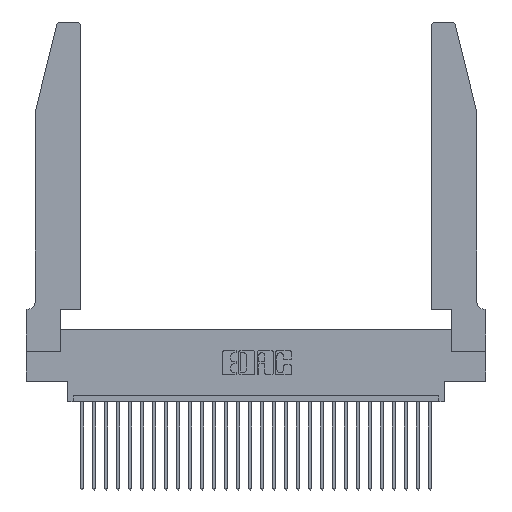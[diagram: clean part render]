
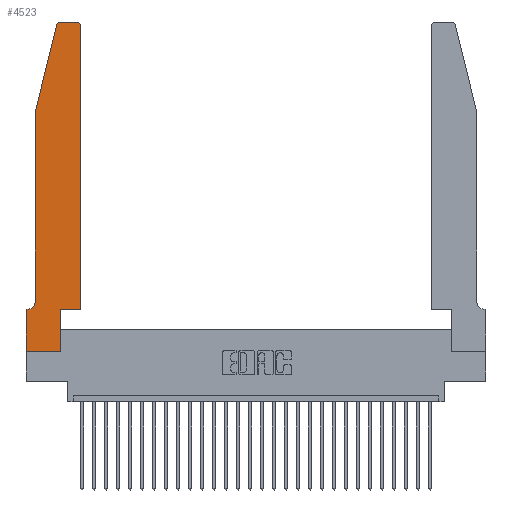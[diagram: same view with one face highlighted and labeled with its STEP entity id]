
A CAD part, top view. The second image highlights one B-rep face of the part: STEP entity #4523.
In plain terms, the highlighted planar face has unit normal (0, 0, 1).
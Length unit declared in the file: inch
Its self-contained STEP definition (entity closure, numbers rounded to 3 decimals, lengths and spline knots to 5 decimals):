
#309 = VECTOR ( 'NONE', #21141, 39.37008 ) ;
#539 = VECTOR ( 'NONE', #13087, 39.37008 ) ;
#681 = DIRECTION ( 'NONE',  ( 1., 0., 0. ) ) ;
#778 = LINE ( 'NONE', #23107, #18697 ) ;
#829 = CARTESIAN_POINT ( 'NONE',  ( 0.0755, 2., 0.37 ) ) ;
#947 = ORIENTED_EDGE ( 'NONE', *, *, #22796, .T. ) ;
#1176 = CARTESIAN_POINT ( 'NONE',  ( 0., 0.35, 0.37 ) ) ;
#1369 = VERTEX_POINT ( 'NONE', #12878 ) ;
#1539 = DIRECTION ( 'NONE',  ( 0., 1., 0. ) ) ;
#2335 = VERTEX_POINT ( 'NONE', #19658 ) ;
#2676 = DIRECTION ( 'NONE',  ( -1., 0., 0. ) ) ;
#2739 = EDGE_CURVE ( 'NONE', #14284, #28371, #19319, .T. ) ;
#2931 = CARTESIAN_POINT ( 'NONE',  ( 0.284, 2.72, 0.37 ) ) ;
#3050 = CARTESIAN_POINT ( 'NONE',  ( 0., 0., 0.37 ) ) ;
#3815 = CIRCLE ( 'NONE', #20481, 0.03 ) ;
#4523 = ADVANCED_FACE ( 'NONE', ( #9105 ), #25926, .T. ) ;
#4568 = ORIENTED_EDGE ( 'NONE', *, *, #15418, .T. ) ;
#4614 = ORIENTED_EDGE ( 'NONE', *, *, #2739, .T. ) ;
#6243 = VERTEX_POINT ( 'NONE', #11317 ) ;
#6420 = CARTESIAN_POINT ( 'NONE',  ( 0., 0., 0.37 ) ) ;
#6519 = LINE ( 'NONE', #12882, #539 ) ;
#6529 = VERTEX_POINT ( 'NONE', #8153 ) ;
#6826 = VERTEX_POINT ( 'NONE', #20742 ) ;
#7390 = DIRECTION ( 'NONE',  ( 0., 1., 0. ) ) ;
#7503 = VECTOR ( 'NONE', #20875, 39.37008 ) ;
#7656 = CIRCLE ( 'NONE', #19356, 0.07 ) ;
#7717 = DIRECTION ( 'NONE',  ( 1., 0., 0. ) ) ;
#8153 = CARTESIAN_POINT ( 'NONE',  ( 0.4505, 0.35, 0.37 ) ) ;
#8216 = DIRECTION ( 'NONE',  ( 0., 0., 1. ) ) ;
#8703 = CARTESIAN_POINT ( 'NONE',  ( 0.2605, 2.75, 0.37 ) ) ;
#9105 = FACE_OUTER_BOUND ( 'NONE', #18436, .T. ) ;
#9528 = EDGE_CURVE ( 'NONE', #6243, #6529, #22151, .T. ) ;
#9641 = EDGE_CURVE ( 'NONE', #1369, #19154, #17126, .T. ) ;
#9747 = ORIENTED_EDGE ( 'NONE', *, *, #21674, .T. ) ;
#9789 = LINE ( 'NONE', #12009, #13646 ) ;
#10173 = CARTESIAN_POINT ( 'NONE',  ( 0.0755, 2., 0.37 ) ) ;
#10863 = ORIENTED_EDGE ( 'NONE', *, *, #9528, .T. ) ;
#10948 = DIRECTION ( 'NONE',  ( -1., 0., 0. ) ) ;
#11317 = CARTESIAN_POINT ( 'NONE',  ( 0.2865, 0.35, 0.37 ) ) ;
#11892 = DIRECTION ( 'NONE',  ( 0., 0., -1. ) ) ;
#11932 = CARTESIAN_POINT ( 'NONE',  ( 0.25487, 2.72718, 0.37 ) ) ;
#12009 = CARTESIAN_POINT ( 'NONE',  ( 0.4505, 0.35, 0.37 ) ) ;
#12341 = DIRECTION ( 'NONE',  ( 1., 0., 0. ) ) ;
#12691 = EDGE_CURVE ( 'NONE', #24017, #6243, #778, .T. ) ;
#12878 = CARTESIAN_POINT ( 'NONE',  ( 0.0055, 0.35, 0.37 ) ) ;
#12882 = CARTESIAN_POINT ( 'NONE',  ( 0., 0., 0.37 ) ) ;
#12885 = AXIS2_PLACEMENT_3D ( 'NONE', #1176, #8216, #12341 ) ;
#13087 = DIRECTION ( 'NONE',  ( 0., -1., 0. ) ) ;
#13646 = VECTOR ( 'NONE', #1539, 39.37008 ) ;
#14089 = AXIS2_PLACEMENT_3D ( 'NONE', #2931, #14109, #681 ) ;
#14109 = DIRECTION ( 'NONE',  ( 0., 0., 1. ) ) ;
#14284 = VERTEX_POINT ( 'NONE', #11932 ) ;
#14329 = DIRECTION ( 'NONE',  ( -1., 0., 0. ) ) ;
#14332 = ORIENTED_EDGE ( 'NONE', *, *, #9641, .T. ) ;
#14447 = EDGE_CURVE ( 'NONE', #6529, #18218, #9789, .T. ) ;
#14870 = ORIENTED_EDGE ( 'NONE', *, *, #15019, .T. ) ;
#15019 = EDGE_CURVE ( 'NONE', #18218, #18714, #3815, .T. ) ;
#15418 = EDGE_CURVE ( 'NONE', #6826, #1369, #7656, .T. ) ;
#15758 = VECTOR ( 'NONE', #21126, 39.37008 ) ;
#15926 = EDGE_CURVE ( 'NONE', #19154, #26882, #6519, .T. ) ;
#17126 = LINE ( 'NONE', #23354, #19647 ) ;
#17622 = ORIENTED_EDGE ( 'NONE', *, *, #12691, .T. ) ;
#18218 = VERTEX_POINT ( 'NONE', #23352 ) ;
#18436 = EDGE_LOOP ( 'NONE', ( #24780, #25961, #4614, #947, #4568, #14332, #27943, #9747, #17622, #10863, #27851, #14870 ) ) ;
#18494 = VECTOR ( 'NONE', #24567, 39.37008 ) ;
#18523 = CARTESIAN_POINT ( 'NONE',  ( 0.2865, 0., 0.37 ) ) ;
#18697 = VECTOR ( 'NONE', #7390, 39.37008 ) ;
#18714 = VERTEX_POINT ( 'NONE', #26429 ) ;
#18752 = CARTESIAN_POINT ( 'NONE',  ( 0.0755, 2., 0.37 ) ) ;
#18909 = EDGE_CURVE ( 'NONE', #2335, #14284, #19736, .T. ) ;
#19154 = VERTEX_POINT ( 'NONE', #21966 ) ;
#19319 = LINE ( 'NONE', #18752, #309 ) ;
#19356 = AXIS2_PLACEMENT_3D ( 'NONE', #25398, #11892, #2676 ) ;
#19647 = VECTOR ( 'NONE', #14329, 39.37008 ) ;
#19658 = CARTESIAN_POINT ( 'NONE',  ( 0.284, 2.75, 0.37 ) ) ;
#19736 = CIRCLE ( 'NONE', #14089, 0.03 ) ;
#20085 = EDGE_CURVE ( 'NONE', #18714, #2335, #20743, .T. ) ;
#20481 = AXIS2_PLACEMENT_3D ( 'NONE', #21064, #27731, #7717 ) ;
#20641 = LINE ( 'NONE', #6420, #18494 ) ;
#20742 = CARTESIAN_POINT ( 'NONE',  ( 0.0755, 0.42, 0.37 ) ) ;
#20743 = LINE ( 'NONE', #8703, #25651 ) ;
#20875 = DIRECTION ( 'NONE',  ( 0., -1., 0. ) ) ;
#21064 = CARTESIAN_POINT ( 'NONE',  ( 0.4205, 2.72, 0.37 ) ) ;
#21126 = DIRECTION ( 'NONE',  ( 1., 0., 0. ) ) ;
#21141 = DIRECTION ( 'NONE',  ( -0.239, -0.971, 0. ) ) ;
#21674 = EDGE_CURVE ( 'NONE', #26882, #24017, #20641, .T. ) ;
#21966 = CARTESIAN_POINT ( 'NONE',  ( 0., 0.35, 0.37 ) ) ;
#22151 = LINE ( 'NONE', #27688, #15758 ) ;
#22796 = EDGE_CURVE ( 'NONE', #28371, #6826, #29020, .T. ) ;
#23107 = CARTESIAN_POINT ( 'NONE',  ( 0.2865, 0.35, 0.37 ) ) ;
#23352 = CARTESIAN_POINT ( 'NONE',  ( 0.4505, 2.72, 0.37 ) ) ;
#23354 = CARTESIAN_POINT ( 'NONE',  ( 0.0755, 0.35, 0.37 ) ) ;
#24017 = VERTEX_POINT ( 'NONE', #18523 ) ;
#24567 = DIRECTION ( 'NONE',  ( 1., 0., 0. ) ) ;
#24780 = ORIENTED_EDGE ( 'NONE', *, *, #20085, .T. ) ;
#25398 = CARTESIAN_POINT ( 'NONE',  ( 0.0055, 0.42, 0.37 ) ) ;
#25651 = VECTOR ( 'NONE', #10948, 39.37008 ) ;
#25926 = PLANE ( 'NONE',  #12885 ) ;
#25961 = ORIENTED_EDGE ( 'NONE', *, *, #18909, .T. ) ;
#26429 = CARTESIAN_POINT ( 'NONE',  ( 0.4205, 2.75, 0.37 ) ) ;
#26882 = VERTEX_POINT ( 'NONE', #3050 ) ;
#27688 = CARTESIAN_POINT ( 'NONE',  ( 0.4505, 0.35, 0.37 ) ) ;
#27731 = DIRECTION ( 'NONE',  ( 0., 0., 1. ) ) ;
#27851 = ORIENTED_EDGE ( 'NONE', *, *, #14447, .T. ) ;
#27943 = ORIENTED_EDGE ( 'NONE', *, *, #15926, .T. ) ;
#28371 = VERTEX_POINT ( 'NONE', #10173 ) ;
#29020 = LINE ( 'NONE', #829, #7503 ) ;
